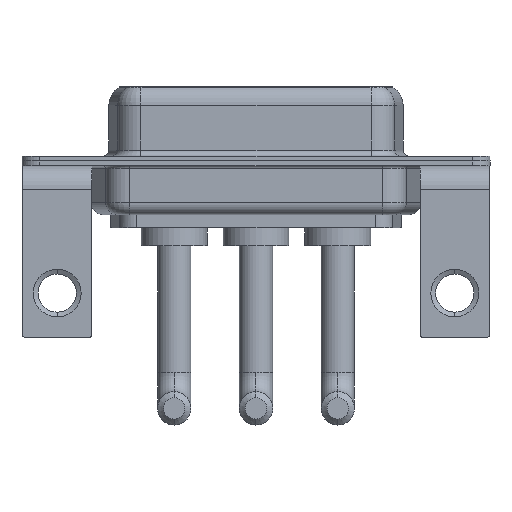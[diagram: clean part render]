
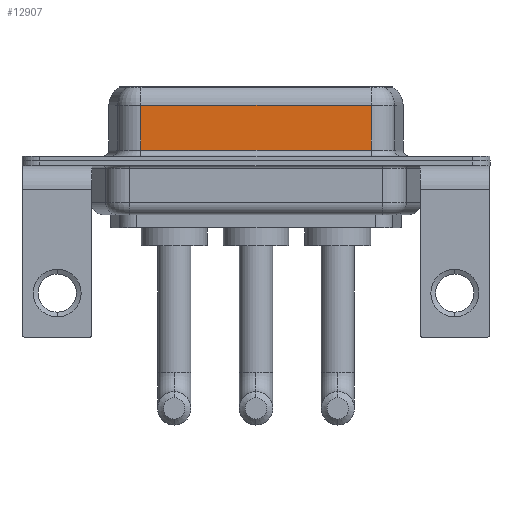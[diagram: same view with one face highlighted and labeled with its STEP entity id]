
A CAD part, front view. The second image highlights one B-rep face of the part: STEP entity #12907.
In plain terms, the highlighted planar face has unit normal (0, -1, 0).
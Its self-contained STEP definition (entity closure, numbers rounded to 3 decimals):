
#98 = LINE ( 'NONE', #10258, #5673 ) ;
#190 = VECTOR ( 'NONE', #2266, 1000. ) ;
#279 = ORIENTED_EDGE ( 'NONE', *, *, #4262, .T. ) ;
#370 = ORIENTED_EDGE ( 'NONE', *, *, #5161, .F. ) ;
#1726 = VERTEX_POINT ( 'NONE', #12861 ) ;
#2266 = DIRECTION ( 'NONE',  ( 0., 0., -1. ) ) ;
#2368 = VERTEX_POINT ( 'NONE', #7603 ) ;
#2403 = DIRECTION ( 'NONE',  ( 0., 0., 1. ) ) ;
#2408 = DIRECTION ( 'NONE',  ( 1., 0., 0. ) ) ;
#2925 = EDGE_CURVE ( 'NONE', #11894, #2368, #7493, .T. ) ;
#3263 = LINE ( 'NONE', #8331, #190 ) ;
#3809 = EDGE_LOOP ( 'NONE', ( #370, #9634, #279, #10437 ) ) ;
#4193 = CARTESIAN_POINT ( 'NONE',  ( 26.287, -3.95, 6.4 ) ) ;
#4262 = EDGE_CURVE ( 'NONE', #5011, #11894, #12499, .T. ) ;
#5011 = VERTEX_POINT ( 'NONE', #7943 ) ;
#5161 = EDGE_CURVE ( 'NONE', #1726, #2368, #3263, .T. ) ;
#5360 = AXIS2_PLACEMENT_3D ( 'NONE', #4193, #10428, #2403 ) ;
#5418 = CARTESIAN_POINT ( 'NONE',  ( 7.013, -3.95, 6.4 ) ) ;
#5673 = VECTOR ( 'NONE', #8234, 1000. ) ;
#6370 = FACE_OUTER_BOUND ( 'NONE', #3809, .T. ) ;
#7493 = LINE ( 'NONE', #11555, #8645 ) ;
#7603 = CARTESIAN_POINT ( 'NONE',  ( 26.287, -3.95, 0.9 ) ) ;
#7943 = CARTESIAN_POINT ( 'NONE',  ( 7.013, -3.95, 4.65 ) ) ;
#8234 = DIRECTION ( 'NONE',  ( -1., 0., 0. ) ) ;
#8331 = CARTESIAN_POINT ( 'NONE',  ( 26.287, -3.95, 6.4 ) ) ;
#8645 = VECTOR ( 'NONE', #2408, 1000. ) ;
#9448 = DIRECTION ( 'NONE',  ( 0., 0., -1. ) ) ;
#9634 = ORIENTED_EDGE ( 'NONE', *, *, #12152, .T. ) ;
#10258 = CARTESIAN_POINT ( 'NONE',  ( 26.287, -3.95, 4.65 ) ) ;
#10428 = DIRECTION ( 'NONE',  ( 0., 1., 0. ) ) ;
#10437 = ORIENTED_EDGE ( 'NONE', *, *, #2925, .T. ) ;
#10958 = VECTOR ( 'NONE', #9448, 1000. ) ;
#11536 = CARTESIAN_POINT ( 'NONE',  ( 7.013, -3.95, 0.9 ) ) ;
#11555 = CARTESIAN_POINT ( 'NONE',  ( 26.287, -3.95, 0.9 ) ) ;
#11894 = VERTEX_POINT ( 'NONE', #11536 ) ;
#12152 = EDGE_CURVE ( 'NONE', #1726, #5011, #98, .T. ) ;
#12404 = PLANE ( 'NONE',  #5360 ) ;
#12499 = LINE ( 'NONE', #5418, #10958 ) ;
#12861 = CARTESIAN_POINT ( 'NONE',  ( 26.287, -3.95, 4.65 ) ) ;
#12907 = ADVANCED_FACE ( 'NONE', ( #6370 ), #12404, .F. ) ;
